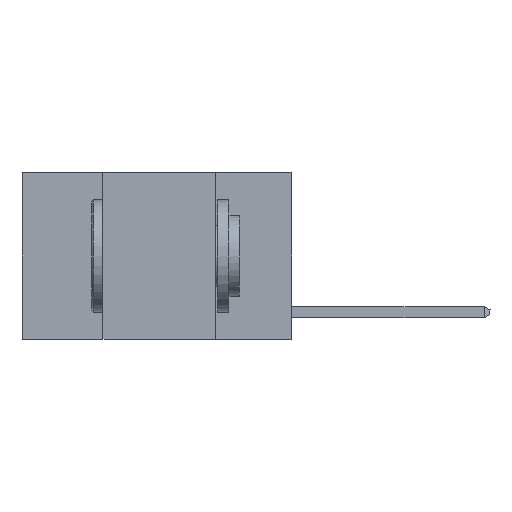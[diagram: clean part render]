
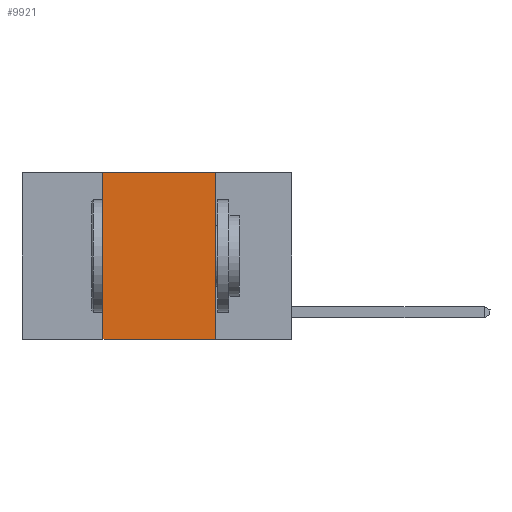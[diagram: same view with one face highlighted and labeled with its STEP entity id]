
A CAD part, left-side view. The second image highlights one B-rep face of the part: STEP entity #9921.
In plain terms, the highlighted planar face has unit normal (-1, 0, 0).
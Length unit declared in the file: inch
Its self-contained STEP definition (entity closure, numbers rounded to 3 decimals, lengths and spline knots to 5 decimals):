
#989 = ORIENTED_EDGE ( 'NONE', *, *, #17638, .F. ) ;
#1122 = VERTEX_POINT ( 'NONE', #16192 ) ;
#1426 = PLANE ( 'NONE',  #11423 ) ;
#2106 = EDGE_CURVE ( 'NONE', #6243, #13062, #8744, .T. ) ;
#3368 = ORIENTED_EDGE ( 'NONE', *, *, #5798, .F. ) ;
#4897 = LINE ( 'NONE', #4984, #13920 ) ;
#4984 = CARTESIAN_POINT ( 'NONE',  ( 0., 0.17, 0. ) ) ;
#5111 = VECTOR ( 'NONE', #6030, 39.37008 ) ;
#5183 = EDGE_CURVE ( 'NONE', #13715, #1122, #17661, .T. ) ;
#5798 = EDGE_CURVE ( 'NONE', #13715, #6243, #15698, .T. ) ;
#6030 = DIRECTION ( 'NONE',  ( 0., 0., 1. ) ) ;
#6243 = VERTEX_POINT ( 'NONE', #11679 ) ;
#8136 = ORIENTED_EDGE ( 'NONE', *, *, #2106, .F. ) ;
#8168 = DIRECTION ( 'NONE',  ( 0., -1., 0. ) ) ;
#8744 = LINE ( 'NONE', #12751, #9923 ) ;
#9921 = ADVANCED_FACE ( 'NONE', ( #10830 ), #1426, .F. ) ;
#9923 = VECTOR ( 'NONE', #14129, 39.37008 ) ;
#10071 = EDGE_LOOP ( 'NONE', ( #989, #8136, #3368, #13437 ) ) ;
#10651 = VECTOR ( 'NONE', #8168, 39.37008 ) ;
#10830 = FACE_OUTER_BOUND ( 'NONE', #10071, .T. ) ;
#11423 = AXIS2_PLACEMENT_3D ( 'NONE', #16390, #12552, #15010 ) ;
#11679 = CARTESIAN_POINT ( 'NONE',  ( 0., 0.42, 0. ) ) ;
#12014 = CARTESIAN_POINT ( 'NONE',  ( 0., 0.6, -0.37 ) ) ;
#12086 = CARTESIAN_POINT ( 'NONE',  ( 0., 0.17, 0. ) ) ;
#12552 = DIRECTION ( 'NONE',  ( 1., 0., 0. ) ) ;
#12560 = CARTESIAN_POINT ( 'NONE',  ( 0., 0.42, -0.37 ) ) ;
#12751 = CARTESIAN_POINT ( 'NONE',  ( 0., 0.6, 0. ) ) ;
#13062 = VERTEX_POINT ( 'NONE', #12086 ) ;
#13437 = ORIENTED_EDGE ( 'NONE', *, *, #5183, .T. ) ;
#13715 = VERTEX_POINT ( 'NONE', #12560 ) ;
#13920 = VECTOR ( 'NONE', #17490, 39.37008 ) ;
#14129 = DIRECTION ( 'NONE',  ( 0., -1., 0. ) ) ;
#15010 = DIRECTION ( 'NONE',  ( 0., 0., -1. ) ) ;
#15698 = LINE ( 'NONE', #15872, #5111 ) ;
#15872 = CARTESIAN_POINT ( 'NONE',  ( 0., 0.42, 0. ) ) ;
#16192 = CARTESIAN_POINT ( 'NONE',  ( 0., 0.17, -0.37 ) ) ;
#16390 = CARTESIAN_POINT ( 'NONE',  ( 0., 0.6, 0. ) ) ;
#17490 = DIRECTION ( 'NONE',  ( 0., 0., -1. ) ) ;
#17638 = EDGE_CURVE ( 'NONE', #13062, #1122, #4897, .T. ) ;
#17661 = LINE ( 'NONE', #12014, #10651 ) ;
